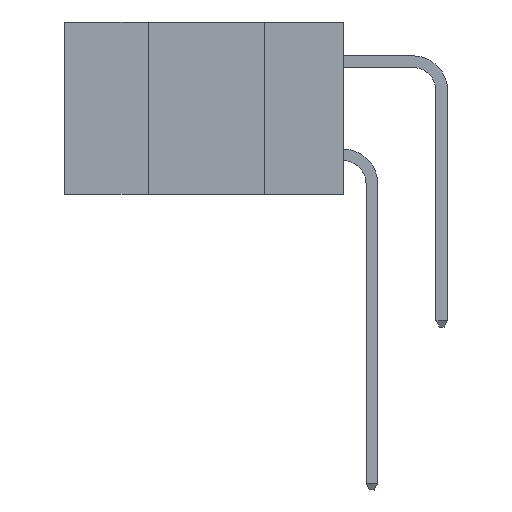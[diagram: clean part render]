
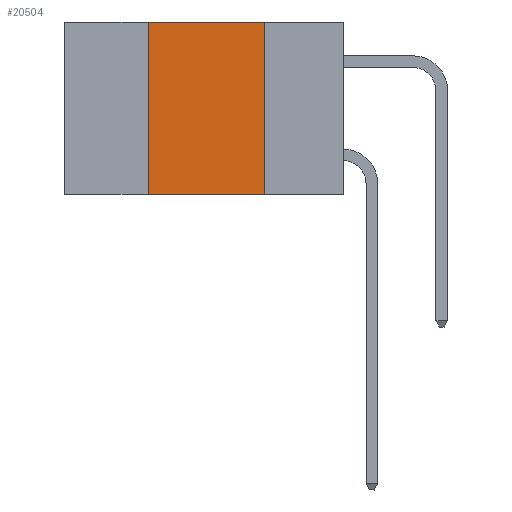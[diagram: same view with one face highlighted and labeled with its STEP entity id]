
A CAD part, left-side view. The second image highlights one B-rep face of the part: STEP entity #20504.
In plain terms, the highlighted planar face has unit normal (-1, 0, 0).
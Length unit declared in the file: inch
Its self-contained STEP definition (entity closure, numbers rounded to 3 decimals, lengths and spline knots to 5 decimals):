
#2457 = LINE ( 'NONE', #18688, #27067 ) ;
#2699 = EDGE_CURVE ( 'NONE', #13045, #15909, #4210, .T. ) ;
#3021 = ORIENTED_EDGE ( 'NONE', *, *, #22667, .F. ) ;
#3341 = EDGE_CURVE ( 'NONE', #4671, #20837, #19075, .T. ) ;
#3646 = CARTESIAN_POINT ( 'NONE',  ( 0., 0.42, 0. ) ) ;
#3765 = ORIENTED_EDGE ( 'NONE', *, *, #2699, .F. ) ;
#3811 = AXIS2_PLACEMENT_3D ( 'NONE', #15007, #5712, #21955 ) ;
#4210 = LINE ( 'NONE', #3646, #28070 ) ;
#4671 = VERTEX_POINT ( 'NONE', #27460 ) ;
#4767 = DIRECTION ( 'NONE',  ( 0., -1., 0. ) ) ;
#5282 = CARTESIAN_POINT ( 'NONE',  ( 0., 0.6, 0. ) ) ;
#5712 = DIRECTION ( 'NONE',  ( 1., 0., 0. ) ) ;
#7097 = EDGE_CURVE ( 'NONE', #13045, #20837, #2457, .T. ) ;
#9950 = DIRECTION ( 'NONE',  ( 0., -1., 0. ) ) ;
#10546 = EDGE_LOOP ( 'NONE', ( #26902, #3021, #3765, #22230 ) ) ;
#13045 = VERTEX_POINT ( 'NONE', #23467 ) ;
#14806 = DIRECTION ( 'NONE',  ( 0., 0., 1. ) ) ;
#15007 = CARTESIAN_POINT ( 'NONE',  ( 0., 0.6, 0. ) ) ;
#15665 = VECTOR ( 'NONE', #9950, 39.37008 ) ;
#15909 = VERTEX_POINT ( 'NONE', #18969 ) ;
#16122 = CARTESIAN_POINT ( 'NONE',  ( 0., 0.17, -0.37 ) ) ;
#18688 = CARTESIAN_POINT ( 'NONE',  ( 0., 0.6, -0.37 ) ) ;
#18969 = CARTESIAN_POINT ( 'NONE',  ( 0., 0.42, 0. ) ) ;
#19075 = LINE ( 'NONE', #20225, #24418 ) ;
#20225 = CARTESIAN_POINT ( 'NONE',  ( 0., 0.17, 0. ) ) ;
#20504 = ADVANCED_FACE ( 'NONE', ( #21384 ), #21861, .F. ) ;
#20629 = DIRECTION ( 'NONE',  ( 0., 0., -1. ) ) ;
#20837 = VERTEX_POINT ( 'NONE', #16122 ) ;
#21384 = FACE_OUTER_BOUND ( 'NONE', #10546, .T. ) ;
#21792 = LINE ( 'NONE', #5282, #15665 ) ;
#21861 = PLANE ( 'NONE',  #3811 ) ;
#21955 = DIRECTION ( 'NONE',  ( 0., 0., -1. ) ) ;
#22230 = ORIENTED_EDGE ( 'NONE', *, *, #7097, .T. ) ;
#22667 = EDGE_CURVE ( 'NONE', #15909, #4671, #21792, .T. ) ;
#23467 = CARTESIAN_POINT ( 'NONE',  ( 0., 0.42, -0.37 ) ) ;
#24418 = VECTOR ( 'NONE', #20629, 39.37008 ) ;
#26902 = ORIENTED_EDGE ( 'NONE', *, *, #3341, .F. ) ;
#27067 = VECTOR ( 'NONE', #4767, 39.37008 ) ;
#27460 = CARTESIAN_POINT ( 'NONE',  ( 0., 0.17, 0. ) ) ;
#28070 = VECTOR ( 'NONE', #14806, 39.37008 ) ;
